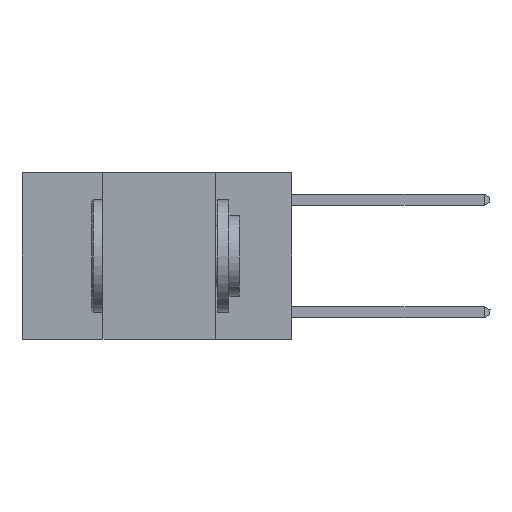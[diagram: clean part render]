
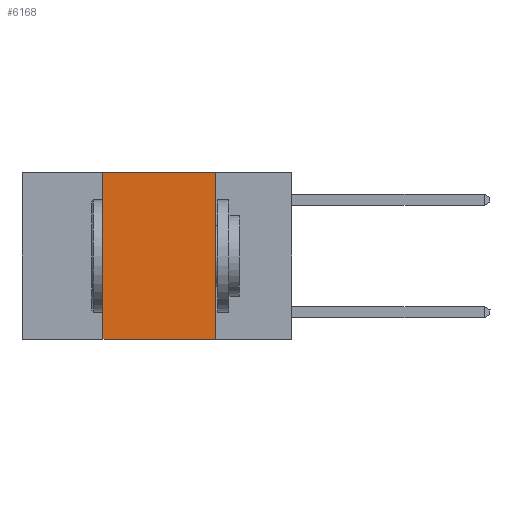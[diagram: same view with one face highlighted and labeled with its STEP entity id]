
A CAD part, left-side view. The second image highlights one B-rep face of the part: STEP entity #6168.
In plain terms, the highlighted planar face has unit normal (-1, 0, 0).
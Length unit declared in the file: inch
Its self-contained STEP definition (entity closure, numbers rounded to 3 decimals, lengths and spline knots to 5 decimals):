
#252 = EDGE_CURVE ( 'NONE', #8666, #1183, #2943, .T. ) ;
#485 = EDGE_CURVE ( 'NONE', #4267, #518, #6234, .T. ) ;
#518 = VERTEX_POINT ( 'NONE', #2994 ) ;
#639 = LINE ( 'NONE', #8313, #4984 ) ;
#975 = ORIENTED_EDGE ( 'NONE', *, *, #9994, .F. ) ;
#1037 = VECTOR ( 'NONE', #3920, 39.37008 ) ;
#1183 = VERTEX_POINT ( 'NONE', #7484 ) ;
#1258 = DIRECTION ( 'NONE',  ( 0., -1., 0. ) ) ;
#2943 = LINE ( 'NONE', #7653, #1037 ) ;
#2994 = CARTESIAN_POINT ( 'NONE',  ( 0., 0.42, 0. ) ) ;
#3116 = CARTESIAN_POINT ( 'NONE',  ( 0., 0.42, -0.37 ) ) ;
#3154 = CARTESIAN_POINT ( 'NONE',  ( 0., 0.42, 0. ) ) ;
#3284 = CARTESIAN_POINT ( 'NONE',  ( 0., 0.17, 0. ) ) ;
#3920 = DIRECTION ( 'NONE',  ( 0., 0., -1. ) ) ;
#4022 = EDGE_CURVE ( 'NONE', #4267, #1183, #6267, .T. ) ;
#4267 = VERTEX_POINT ( 'NONE', #3116 ) ;
#4912 = DIRECTION ( 'NONE',  ( 0., 0., 1. ) ) ;
#4984 = VECTOR ( 'NONE', #9099, 39.37008 ) ;
#5055 = CARTESIAN_POINT ( 'NONE',  ( 0., 0.6, 0. ) ) ;
#5093 = DIRECTION ( 'NONE',  ( 0., 0., -1. ) ) ;
#5275 = ORIENTED_EDGE ( 'NONE', *, *, #485, .F. ) ;
#6096 = CARTESIAN_POINT ( 'NONE',  ( 0., 0.6, -0.37 ) ) ;
#6168 = ADVANCED_FACE ( 'NONE', ( #6439 ), #9014, .F. ) ;
#6234 = LINE ( 'NONE', #3154, #6479 ) ;
#6267 = LINE ( 'NONE', #6096, #10426 ) ;
#6439 = FACE_OUTER_BOUND ( 'NONE', #9913, .T. ) ;
#6479 = VECTOR ( 'NONE', #4912, 39.37008 ) ;
#7113 = AXIS2_PLACEMENT_3D ( 'NONE', #5055, #9803, #5093 ) ;
#7368 = ORIENTED_EDGE ( 'NONE', *, *, #4022, .T. ) ;
#7484 = CARTESIAN_POINT ( 'NONE',  ( 0., 0.17, -0.37 ) ) ;
#7653 = CARTESIAN_POINT ( 'NONE',  ( 0., 0.17, 0. ) ) ;
#8313 = CARTESIAN_POINT ( 'NONE',  ( 0., 0.6, 0. ) ) ;
#8666 = VERTEX_POINT ( 'NONE', #3284 ) ;
#9014 = PLANE ( 'NONE',  #7113 ) ;
#9099 = DIRECTION ( 'NONE',  ( 0., -1., 0. ) ) ;
#9220 = ORIENTED_EDGE ( 'NONE', *, *, #252, .F. ) ;
#9803 = DIRECTION ( 'NONE',  ( 1., 0., 0. ) ) ;
#9913 = EDGE_LOOP ( 'NONE', ( #9220, #975, #5275, #7368 ) ) ;
#9994 = EDGE_CURVE ( 'NONE', #518, #8666, #639, .T. ) ;
#10426 = VECTOR ( 'NONE', #1258, 39.37008 ) ;
